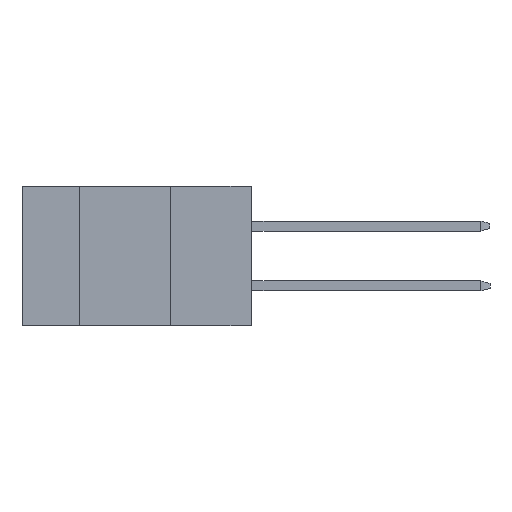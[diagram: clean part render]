
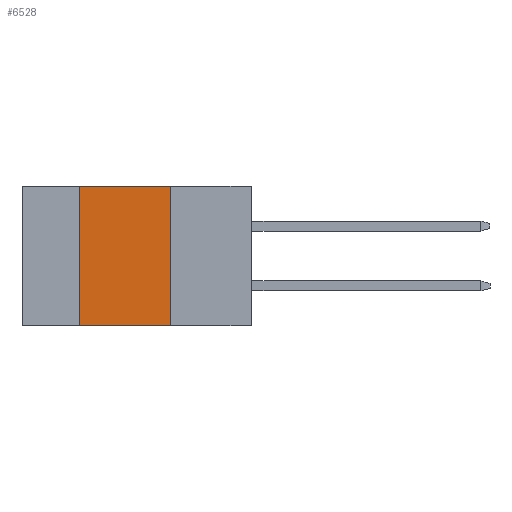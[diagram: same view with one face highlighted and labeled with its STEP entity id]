
A CAD part, left-side view. The second image highlights one B-rep face of the part: STEP entity #6528.
In plain terms, the highlighted planar face has unit normal (-1, 0, 0).
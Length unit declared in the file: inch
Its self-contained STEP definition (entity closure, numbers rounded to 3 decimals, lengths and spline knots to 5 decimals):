
#55 = DIRECTION ( 'NONE',  ( 0., -1., 0. ) ) ;
#491 = VERTEX_POINT ( 'NONE', #17051 ) ;
#1518 = PLANE ( 'NONE',  #5645 ) ;
#1573 = VERTEX_POINT ( 'NONE', #5666 ) ;
#1921 = EDGE_CURVE ( 'NONE', #17450, #491, #4975, .T. ) ;
#2198 = EDGE_CURVE ( 'NONE', #4254, #1573, #5636, .T. ) ;
#2517 = LINE ( 'NONE', #16088, #17791 ) ;
#3881 = CARTESIAN_POINT ( 'NONE',  ( 0., 0.54, -0.437 ) ) ;
#4220 = ORIENTED_EDGE ( 'NONE', *, *, #2198, .T. ) ;
#4254 = VERTEX_POINT ( 'NONE', #3881 ) ;
#4359 = EDGE_CURVE ( 'NONE', #4254, #17450, #2517, .T. ) ;
#4759 = DIRECTION ( 'NONE',  ( 1., 0., 0. ) ) ;
#4975 = LINE ( 'NONE', #21768, #21195 ) ;
#5636 = LINE ( 'NONE', #12423, #14132 ) ;
#5645 = AXIS2_PLACEMENT_3D ( 'NONE', #11523, #4759, #10081 ) ;
#5666 = CARTESIAN_POINT ( 'NONE',  ( 0., 0.254, -0.437 ) ) ;
#6528 = ADVANCED_FACE ( 'NONE', ( #19889 ), #1518, .F. ) ;
#7232 = CARTESIAN_POINT ( 'NONE',  ( 0., 0.54, 0. ) ) ;
#9089 = CARTESIAN_POINT ( 'NONE',  ( 0., 0.254, -0.437 ) ) ;
#9210 = LINE ( 'NONE', #9089, #17860 ) ;
#9362 = ORIENTED_EDGE ( 'NONE', *, *, #18114, .F. ) ;
#9531 = EDGE_LOOP ( 'NONE', ( #9362, #12090, #15279, #4220 ) ) ;
#10081 = DIRECTION ( 'NONE',  ( 0., 0., -1. ) ) ;
#11523 = CARTESIAN_POINT ( 'NONE',  ( 0., 0.72, 0. ) ) ;
#12090 = ORIENTED_EDGE ( 'NONE', *, *, #1921, .F. ) ;
#12423 = CARTESIAN_POINT ( 'NONE',  ( 0., 0.72, -0.437 ) ) ;
#14132 = VECTOR ( 'NONE', #55, 39.37008 ) ;
#15279 = ORIENTED_EDGE ( 'NONE', *, *, #4359, .F. ) ;
#15891 = DIRECTION ( 'NONE',  ( 0., 0., -1. ) ) ;
#16088 = CARTESIAN_POINT ( 'NONE',  ( 0., 0.54, -0.437 ) ) ;
#16412 = DIRECTION ( 'NONE',  ( 0., -1., 0. ) ) ;
#17051 = CARTESIAN_POINT ( 'NONE',  ( 0., 0.254, 0. ) ) ;
#17450 = VERTEX_POINT ( 'NONE', #7232 ) ;
#17791 = VECTOR ( 'NONE', #19638, 39.37008 ) ;
#17860 = VECTOR ( 'NONE', #15891, 39.37008 ) ;
#18114 = EDGE_CURVE ( 'NONE', #491, #1573, #9210, .T. ) ;
#19638 = DIRECTION ( 'NONE',  ( 0., 0., 1. ) ) ;
#19889 = FACE_OUTER_BOUND ( 'NONE', #9531, .T. ) ;
#21195 = VECTOR ( 'NONE', #16412, 39.37008 ) ;
#21768 = CARTESIAN_POINT ( 'NONE',  ( 0., 0.72, 0. ) ) ;
